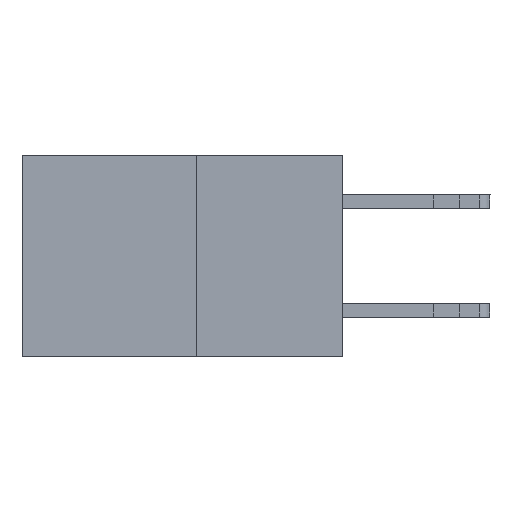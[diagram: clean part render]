
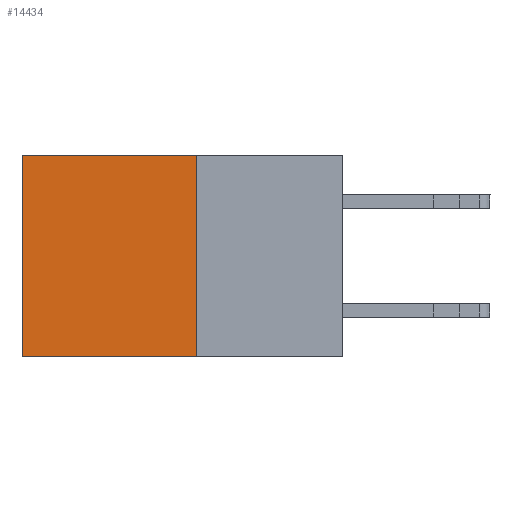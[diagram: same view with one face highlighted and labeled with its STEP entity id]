
A CAD part, left-side view. The second image highlights one B-rep face of the part: STEP entity #14434.
In plain terms, the highlighted planar face has unit normal (-1, 0, 0).
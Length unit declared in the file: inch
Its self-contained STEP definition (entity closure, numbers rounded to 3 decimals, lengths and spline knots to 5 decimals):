
#231 = CARTESIAN_POINT ( 'NONE',  ( 0.277, 0.27, -0.37 ) ) ;
#330 = AXIS2_PLACEMENT_3D ( 'NONE', #8813, #14262, #3590 ) ;
#1099 = EDGE_CURVE ( 'NONE', #14377, #1341, #11800, .T. ) ;
#1341 = VERTEX_POINT ( 'NONE', #10562 ) ;
#1631 = ORIENTED_EDGE ( 'NONE', *, *, #10985, .T. ) ;
#2026 = DIRECTION ( 'NONE',  ( 0., 1., 0. ) ) ;
#2489 = EDGE_CURVE ( 'NONE', #14377, #12796, #4428, .T. ) ;
#2896 = DIRECTION ( 'NONE',  ( 0., 0., -1. ) ) ;
#3590 = DIRECTION ( 'NONE',  ( 0., 0., -1. ) ) ;
#3841 = VECTOR ( 'NONE', #7248, 39.37008 ) ;
#4428 = LINE ( 'NONE', #231, #13048 ) ;
#4546 = CARTESIAN_POINT ( 'NONE',  ( 0.277, 0.59, -0.37 ) ) ;
#5507 = VECTOR ( 'NONE', #15780, 39.37008 ) ;
#5898 = CARTESIAN_POINT ( 'NONE',  ( 0.277, 0.27, -0.37 ) ) ;
#7248 = DIRECTION ( 'NONE',  ( 0., 0., -1. ) ) ;
#8283 = CARTESIAN_POINT ( 'NONE',  ( 0.277, 0.27, 0. ) ) ;
#8535 = EDGE_CURVE ( 'NONE', #12796, #16649, #10188, .T. ) ;
#8813 = CARTESIAN_POINT ( 'NONE',  ( 0.277, 0.27, -0.37 ) ) ;
#10188 = LINE ( 'NONE', #5898, #10621 ) ;
#10562 = CARTESIAN_POINT ( 'NONE',  ( 0.277, 0.59, 0. ) ) ;
#10621 = VECTOR ( 'NONE', #2026, 39.37008 ) ;
#10985 = EDGE_CURVE ( 'NONE', #1341, #16649, #16745, .T. ) ;
#11291 = ORIENTED_EDGE ( 'NONE', *, *, #2489, .F. ) ;
#11800 = LINE ( 'NONE', #8283, #5507 ) ;
#11974 = CARTESIAN_POINT ( 'NONE',  ( 0.277, 0.59, -0.37 ) ) ;
#12666 = CARTESIAN_POINT ( 'NONE',  ( 0.277, 0.27, -0.37 ) ) ;
#12731 = ORIENTED_EDGE ( 'NONE', *, *, #1099, .T. ) ;
#12796 = VERTEX_POINT ( 'NONE', #12666 ) ;
#13048 = VECTOR ( 'NONE', #2896, 39.37008 ) ;
#13087 = PLANE ( 'NONE',  #330 ) ;
#13726 = EDGE_LOOP ( 'NONE', ( #1631, #15014, #11291, #12731 ) ) ;
#14262 = DIRECTION ( 'NONE',  ( 1., 0., 0. ) ) ;
#14377 = VERTEX_POINT ( 'NONE', #16731 ) ;
#14434 = ADVANCED_FACE ( 'NONE', ( #17226 ), #13087, .F. ) ;
#15014 = ORIENTED_EDGE ( 'NONE', *, *, #8535, .F. ) ;
#15780 = DIRECTION ( 'NONE',  ( 0., 1., 0. ) ) ;
#16649 = VERTEX_POINT ( 'NONE', #11974 ) ;
#16731 = CARTESIAN_POINT ( 'NONE',  ( 0.277, 0.27, 0. ) ) ;
#16745 = LINE ( 'NONE', #4546, #3841 ) ;
#17226 = FACE_OUTER_BOUND ( 'NONE', #13726, .T. ) ;
